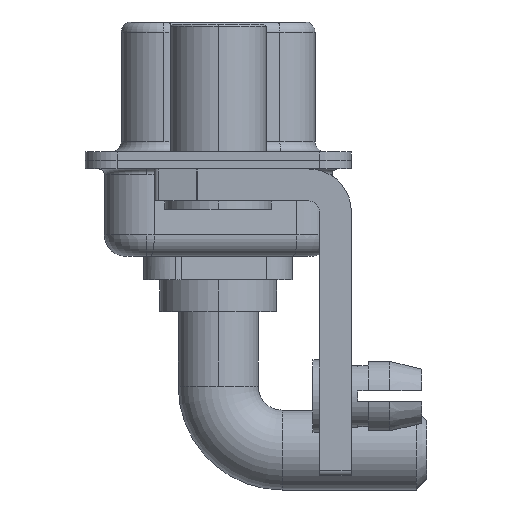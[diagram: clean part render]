
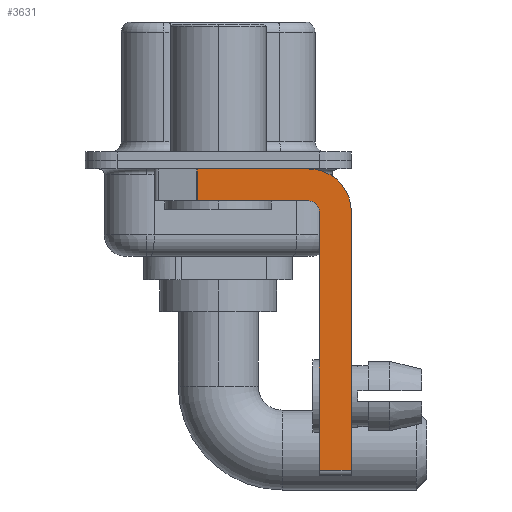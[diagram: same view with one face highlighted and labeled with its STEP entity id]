
A CAD part, left-side view. The second image highlights one B-rep face of the part: STEP entity #3631.
In plain terms, the highlighted planar face has unit normal (-1, 0, 0).
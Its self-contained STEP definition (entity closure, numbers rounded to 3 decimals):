
#90 = CARTESIAN_POINT ( 'NONE',  ( -2.9, -6.25, -14.55 ) ) ;
#575 = DIRECTION ( 'NONE',  ( 0., 1., 0. ) ) ;
#867 = VECTOR ( 'NONE', #575, 1000. ) ;
#1359 = LINE ( 'NONE', #8016, #11753 ) ;
#1563 = DIRECTION ( 'NONE',  ( -1., 0., 0. ) ) ;
#1661 = DIRECTION ( 'NONE',  ( 0., 0., 1. ) ) ;
#1968 = DIRECTION ( 'NONE',  ( 1., 0., 0. ) ) ;
#2316 = ORIENTED_EDGE ( 'NONE', *, *, #9496, .F. ) ;
#2451 = EDGE_CURVE ( 'NONE', #17425, #12178, #5403, .T. ) ;
#2577 = VERTEX_POINT ( 'NONE', #16005 ) ;
#2789 = CIRCLE ( 'NONE', #6829, 2. ) ;
#3425 = VERTEX_POINT ( 'NONE', #14240 ) ;
#3497 = VERTEX_POINT ( 'NONE', #8888 ) ;
#3611 = VERTEX_POINT ( 'NONE', #5051 ) ;
#3631 = ADVANCED_FACE ( 'NONE', ( #12036 ), #15020, .F. ) ;
#4127 = DIRECTION ( 'NONE',  ( 0., 0., 1. ) ) ;
#4194 = DIRECTION ( 'NONE',  ( 0., 0., -1. ) ) ;
#4399 = VECTOR ( 'NONE', #6989, 1000. ) ;
#4478 = CARTESIAN_POINT ( 'NONE',  ( -2.9, -4.25, -2.4 ) ) ;
#4723 = ORIENTED_EDGE ( 'NONE', *, *, #2451, .F. ) ;
#5051 = CARTESIAN_POINT ( 'NONE',  ( -2.9, 0.978, -1.9 ) ) ;
#5141 = DIRECTION ( 'NONE',  ( 1., 0., 0. ) ) ;
#5403 = CIRCLE ( 'NONE', #15267, 0.5 ) ;
#5622 = CARTESIAN_POINT ( 'NONE',  ( -2.9, -4.25, -14.55 ) ) ;
#5722 = LINE ( 'NONE', #5622, #4399 ) ;
#5740 = EDGE_CURVE ( 'NONE', #3425, #2577, #2789, .T. ) ;
#5796 = VERTEX_POINT ( 'NONE', #15944 ) ;
#6099 = AXIS2_PLACEMENT_3D ( 'NONE', #17567, #5141, #16226 ) ;
#6409 = ORIENTED_EDGE ( 'NONE', *, *, #8617, .F. ) ;
#6470 = ORIENTED_EDGE ( 'NONE', *, *, #17691, .T. ) ;
#6829 = AXIS2_PLACEMENT_3D ( 'NONE', #7599, #1968, #8966 ) ;
#6989 = DIRECTION ( 'NONE',  ( 0., -1., 0. ) ) ;
#7012 = CARTESIAN_POINT ( 'NONE',  ( -2.9, -6.25, -2.4 ) ) ;
#7599 = CARTESIAN_POINT ( 'NONE',  ( -2.9, -4.25, -2.4 ) ) ;
#7659 = LINE ( 'NONE', #16006, #867 ) ;
#8016 = CARTESIAN_POINT ( 'NONE',  ( -2.9, 0.978, -1.9 ) ) ;
#8102 = DIRECTION ( 'NONE',  ( 0., 0., -1. ) ) ;
#8418 = CARTESIAN_POINT ( 'NONE',  ( -2.9, -4.75, -14.8 ) ) ;
#8617 = EDGE_CURVE ( 'NONE', #3497, #17425, #10944, .T. ) ;
#8888 = CARTESIAN_POINT ( 'NONE',  ( -2.9, -4.75, -14.55 ) ) ;
#8966 = DIRECTION ( 'NONE',  ( 0., 0., -1. ) ) ;
#9467 = CARTESIAN_POINT ( 'NONE',  ( -2.9, -4.25, -1.9 ) ) ;
#9496 = EDGE_CURVE ( 'NONE', #12178, #3611, #7659, .T. ) ;
#9736 = LINE ( 'NONE', #7012, #15709 ) ;
#9793 = VERTEX_POINT ( 'NONE', #90 ) ;
#9984 = ORIENTED_EDGE ( 'NONE', *, *, #12320, .F. ) ;
#10322 = EDGE_LOOP ( 'NONE', ( #11878, #6470, #2316, #4723, #6409, #13250, #9984, #17333 ) ) ;
#10944 = LINE ( 'NONE', #8418, #17942 ) ;
#11180 = VECTOR ( 'NONE', #12958, 1000. ) ;
#11593 = CARTESIAN_POINT ( 'NONE',  ( -2.9, 3., -0.4 ) ) ;
#11753 = VECTOR ( 'NONE', #8102, 1000. ) ;
#11878 = ORIENTED_EDGE ( 'NONE', *, *, #15881, .F. ) ;
#12036 = FACE_OUTER_BOUND ( 'NONE', #10322, .T. ) ;
#12178 = VERTEX_POINT ( 'NONE', #9467 ) ;
#12320 = EDGE_CURVE ( 'NONE', #2577, #9793, #9736, .T. ) ;
#12770 = EDGE_CURVE ( 'NONE', #3497, #9793, #5722, .T. ) ;
#12958 = DIRECTION ( 'NONE',  ( 0., -1., 0. ) ) ;
#13250 = ORIENTED_EDGE ( 'NONE', *, *, #12770, .T. ) ;
#13319 = LINE ( 'NONE', #11593, #11180 ) ;
#14240 = CARTESIAN_POINT ( 'NONE',  ( -2.9, -4.25, -0.4 ) ) ;
#15020 = PLANE ( 'NONE',  #6099 ) ;
#15267 = AXIS2_PLACEMENT_3D ( 'NONE', #4478, #1563, #1661 ) ;
#15558 = CARTESIAN_POINT ( 'NONE',  ( -2.9, -4.75, -2.4 ) ) ;
#15709 = VECTOR ( 'NONE', #4194, 1000. ) ;
#15881 = EDGE_CURVE ( 'NONE', #5796, #3425, #13319, .T. ) ;
#15944 = CARTESIAN_POINT ( 'NONE',  ( -2.9, 0.978, -0.4 ) ) ;
#16005 = CARTESIAN_POINT ( 'NONE',  ( -2.9, -6.25, -2.4 ) ) ;
#16006 = CARTESIAN_POINT ( 'NONE',  ( -2.9, -4.25, -1.9 ) ) ;
#16226 = DIRECTION ( 'NONE',  ( 0., 0., -1. ) ) ;
#17333 = ORIENTED_EDGE ( 'NONE', *, *, #5740, .F. ) ;
#17425 = VERTEX_POINT ( 'NONE', #15558 ) ;
#17567 = CARTESIAN_POINT ( 'NONE',  ( -2.9, -4.25, -2.4 ) ) ;
#17691 = EDGE_CURVE ( 'NONE', #5796, #3611, #1359, .T. ) ;
#17942 = VECTOR ( 'NONE', #4127, 1000. ) ;
